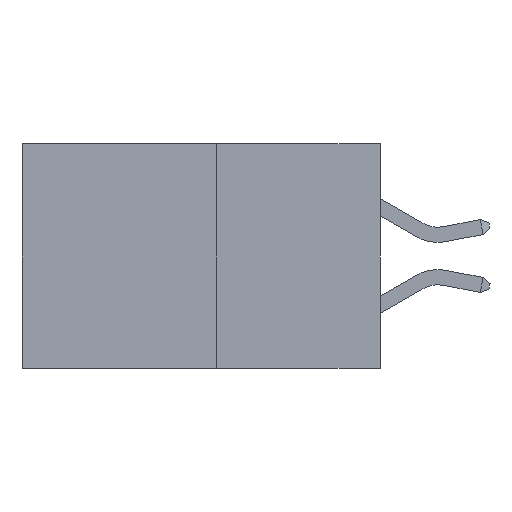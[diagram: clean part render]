
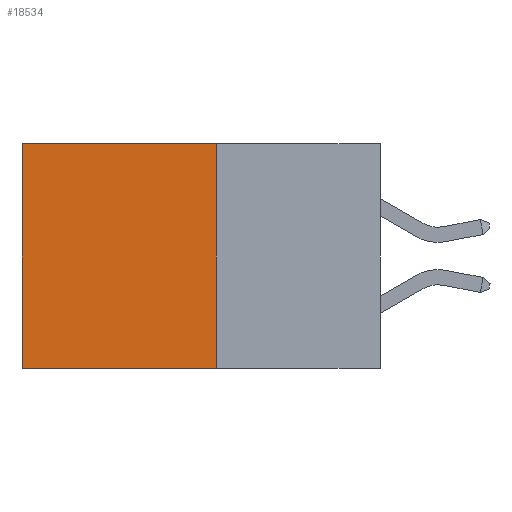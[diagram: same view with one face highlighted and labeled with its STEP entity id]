
A CAD part, left-side view. The second image highlights one B-rep face of the part: STEP entity #18534.
In plain terms, the highlighted planar face has unit normal (-1, 0, 0).
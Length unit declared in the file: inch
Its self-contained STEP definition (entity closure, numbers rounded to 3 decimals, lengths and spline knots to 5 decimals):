
#399 = EDGE_CURVE ( 'NONE', #28738, #5238, #4916, .T. ) ;
#1852 = DIRECTION ( 'NONE',  ( 0., 0., -1. ) ) ;
#1994 = AXIS2_PLACEMENT_3D ( 'NONE', #8220, #10911, #29472 ) ;
#2338 = VECTOR ( 'NONE', #22171, 39.37008 ) ;
#4916 = LINE ( 'NONE', #20413, #5767 ) ;
#5238 = VERTEX_POINT ( 'NONE', #33135 ) ;
#5494 = PLANE ( 'NONE',  #1994 ) ;
#5767 = VECTOR ( 'NONE', #8320, 39.37008 ) ;
#7172 = VECTOR ( 'NONE', #26338, 39.37008 ) ;
#7702 = CARTESIAN_POINT ( 'NONE',  ( 0.277, 0.27, -0.37 ) ) ;
#7992 = CARTESIAN_POINT ( 'NONE',  ( 0.277, 0.27, -0.37 ) ) ;
#8219 = CARTESIAN_POINT ( 'NONE',  ( 0.277, 0.27, 0. ) ) ;
#8220 = CARTESIAN_POINT ( 'NONE',  ( 0.277, 0.27, -0.37 ) ) ;
#8320 = DIRECTION ( 'NONE',  ( 0., 1., 0. ) ) ;
#9799 = EDGE_CURVE ( 'NONE', #25226, #14535, #19686, .T. ) ;
#10911 = DIRECTION ( 'NONE',  ( 1., 0., 0. ) ) ;
#10916 = ORIENTED_EDGE ( 'NONE', *, *, #9799, .F. ) ;
#13761 = FACE_OUTER_BOUND ( 'NONE', #18598, .T. ) ;
#14535 = VERTEX_POINT ( 'NONE', #26531 ) ;
#15782 = VECTOR ( 'NONE', #1852, 39.37008 ) ;
#16649 = LINE ( 'NONE', #19501, #2338 ) ;
#18534 = ADVANCED_FACE ( 'NONE', ( #13761 ), #5494, .F. ) ;
#18598 = EDGE_LOOP ( 'NONE', ( #24283, #10916, #33313, #26216 ) ) ;
#19501 = CARTESIAN_POINT ( 'NONE',  ( 0.277, 0.59, -0.37 ) ) ;
#19686 = LINE ( 'NONE', #7702, #7172 ) ;
#20413 = CARTESIAN_POINT ( 'NONE',  ( 0.277, 0.27, 0. ) ) ;
#22171 = DIRECTION ( 'NONE',  ( 0., 0., -1. ) ) ;
#23632 = LINE ( 'NONE', #33704, #15782 ) ;
#24283 = ORIENTED_EDGE ( 'NONE', *, *, #28884, .T. ) ;
#25226 = VERTEX_POINT ( 'NONE', #7992 ) ;
#26216 = ORIENTED_EDGE ( 'NONE', *, *, #399, .T. ) ;
#26338 = DIRECTION ( 'NONE',  ( 0., 1., 0. ) ) ;
#26531 = CARTESIAN_POINT ( 'NONE',  ( 0.277, 0.59, -0.37 ) ) ;
#28738 = VERTEX_POINT ( 'NONE', #8219 ) ;
#28884 = EDGE_CURVE ( 'NONE', #5238, #14535, #16649, .T. ) ;
#29472 = DIRECTION ( 'NONE',  ( 0., 0., -1. ) ) ;
#33135 = CARTESIAN_POINT ( 'NONE',  ( 0.277, 0.59, 0. ) ) ;
#33313 = ORIENTED_EDGE ( 'NONE', *, *, #34046, .F. ) ;
#33704 = CARTESIAN_POINT ( 'NONE',  ( 0.277, 0.27, -0.37 ) ) ;
#34046 = EDGE_CURVE ( 'NONE', #28738, #25226, #23632, .T. ) ;
